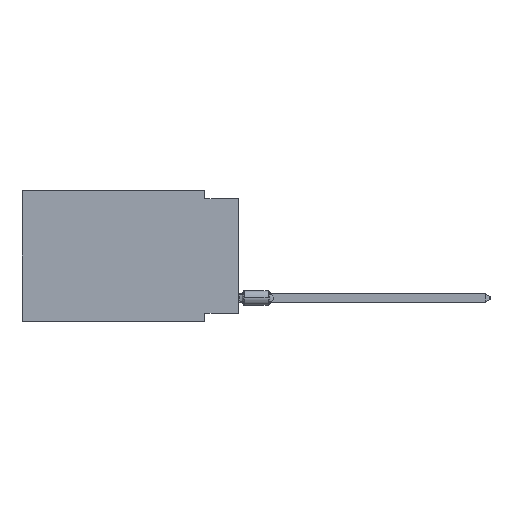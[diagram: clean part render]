
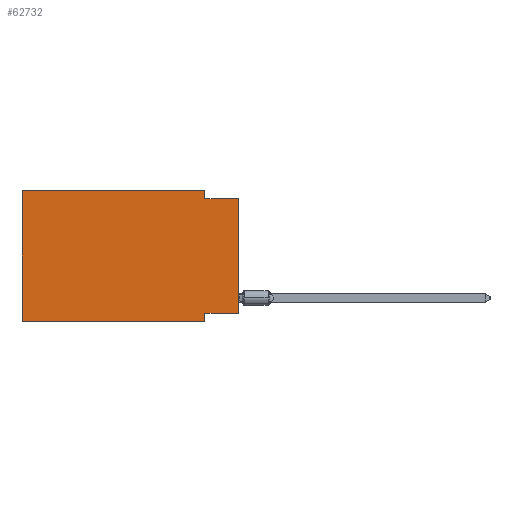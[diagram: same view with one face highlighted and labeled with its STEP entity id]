
A CAD part, left-side view. The second image highlights one B-rep face of the part: STEP entity #62732.
In plain terms, the highlighted planar face has unit normal (-1, 0, 0).
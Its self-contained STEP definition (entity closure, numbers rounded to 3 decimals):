
#473 = ORIENTED_EDGE ( 'NONE', *, *, #65297, .F. ) ;
#792 = CARTESIAN_POINT ( 'NONE',  ( 0., 0., -9.271 ) ) ;
#1288 = VERTEX_POINT ( 'NONE', #24832 ) ;
#1534 = ORIENTED_EDGE ( 'NONE', *, *, #37827, .F. ) ;
#1687 = VERTEX_POINT ( 'NONE', #4763 ) ;
#1880 = DIRECTION ( 'NONE',  ( 0., 0., 1. ) ) ;
#2244 = DIRECTION ( 'NONE',  ( 0., 0., -1. ) ) ;
#4738 = DIRECTION ( 'NONE',  ( 0., -1., 0. ) ) ;
#4763 = CARTESIAN_POINT ( 'NONE',  ( 0., 2.54, -0.635 ) ) ;
#4782 = VERTEX_POINT ( 'NONE', #67174 ) ;
#5969 = ORIENTED_EDGE ( 'NONE', *, *, #32607, .T. ) ;
#6378 = EDGE_LOOP ( 'NONE', ( #5969, #16772, #473, #15447, #13723, #21417, #56265, #1534 ) ) ;
#6649 = CARTESIAN_POINT ( 'NONE',  ( 0., 2.54, -9.906 ) ) ;
#7434 = DIRECTION ( 'NONE',  ( 0., -1., 0. ) ) ;
#8665 = VECTOR ( 'NONE', #42548, 1000. ) ;
#11778 = CARTESIAN_POINT ( 'NONE',  ( 0., 16.383, 0. ) ) ;
#12164 = PLANE ( 'NONE',  #34855 ) ;
#13723 = ORIENTED_EDGE ( 'NONE', *, *, #46928, .F. ) ;
#15167 = VECTOR ( 'NONE', #37014, 1000. ) ;
#15447 = ORIENTED_EDGE ( 'NONE', *, *, #65070, .F. ) ;
#15484 = CARTESIAN_POINT ( 'NONE',  ( 0., 16.383, 0. ) ) ;
#16772 = ORIENTED_EDGE ( 'NONE', *, *, #66112, .F. ) ;
#18406 = CARTESIAN_POINT ( 'NONE',  ( 0., 0., -0.635 ) ) ;
#18511 = CARTESIAN_POINT ( 'NONE',  ( 0., 2.54, 0. ) ) ;
#18996 = LINE ( 'NONE', #29242, #35188 ) ;
#19746 = CARTESIAN_POINT ( 'NONE',  ( 0., 16.383, -9.906 ) ) ;
#20221 = VECTOR ( 'NONE', #29838, 1000. ) ;
#21287 = VECTOR ( 'NONE', #4738, 1000. ) ;
#21417 = ORIENTED_EDGE ( 'NONE', *, *, #29095, .T. ) ;
#22633 = DIRECTION ( 'NONE',  ( 0., 0., -1. ) ) ;
#24391 = VERTEX_POINT ( 'NONE', #53255 ) ;
#24832 = CARTESIAN_POINT ( 'NONE',  ( 0., 16.383, 0. ) ) ;
#25863 = VECTOR ( 'NONE', #7434, 1000. ) ;
#29095 = EDGE_CURVE ( 'NONE', #24391, #58233, #66915, .T. ) ;
#29242 = CARTESIAN_POINT ( 'NONE',  ( 0., 0., -9.271 ) ) ;
#29838 = DIRECTION ( 'NONE',  ( 0., -1., 0. ) ) ;
#32607 = EDGE_CURVE ( 'NONE', #60291, #63623, #62307, .T. ) ;
#34855 = AXIS2_PLACEMENT_3D ( 'NONE', #59305, #53158, #2244 ) ;
#35188 = VECTOR ( 'NONE', #67162, 1000. ) ;
#37014 = DIRECTION ( 'NONE',  ( 0., 0., 1. ) ) ;
#37079 = LINE ( 'NONE', #11778, #43969 ) ;
#37827 = EDGE_CURVE ( 'NONE', #60291, #51407, #18996, .T. ) ;
#42548 = DIRECTION ( 'NONE',  ( 0., 0., -1. ) ) ;
#43586 = FACE_OUTER_BOUND ( 'NONE', #6378, .T. ) ;
#43661 = CARTESIAN_POINT ( 'NONE',  ( 0., 0., -0.635 ) ) ;
#43969 = VECTOR ( 'NONE', #1880, 1000. ) ;
#46928 = EDGE_CURVE ( 'NONE', #24391, #1288, #37079, .T. ) ;
#49463 = LINE ( 'NONE', #43661, #25863 ) ;
#51407 = VERTEX_POINT ( 'NONE', #59390 ) ;
#52455 = LINE ( 'NONE', #57575, #8665 ) ;
#53158 = DIRECTION ( 'NONE',  ( 1., 0., 0. ) ) ;
#53255 = CARTESIAN_POINT ( 'NONE',  ( 0., 16.383, -9.906 ) ) ;
#56265 = ORIENTED_EDGE ( 'NONE', *, *, #67474, .F. ) ;
#57575 = CARTESIAN_POINT ( 'NONE',  ( 0., 2.54, -9.906 ) ) ;
#58233 = VERTEX_POINT ( 'NONE', #6649 ) ;
#59305 = CARTESIAN_POINT ( 'NONE',  ( 0., 16.383, 0. ) ) ;
#59390 = CARTESIAN_POINT ( 'NONE',  ( 0., 2.54, -9.271 ) ) ;
#60291 = VERTEX_POINT ( 'NONE', #792 ) ;
#62307 = LINE ( 'NONE', #67104, #15167 ) ;
#62732 = ADVANCED_FACE ( 'NONE', ( #43586 ), #12164, .F. ) ;
#63623 = VERTEX_POINT ( 'NONE', #18406 ) ;
#64339 = LINE ( 'NONE', #18511, #66085 ) ;
#65070 = EDGE_CURVE ( 'NONE', #1288, #4782, #66080, .T. ) ;
#65297 = EDGE_CURVE ( 'NONE', #4782, #1687, #64339, .T. ) ;
#66080 = LINE ( 'NONE', #15484, #20221 ) ;
#66085 = VECTOR ( 'NONE', #22633, 1000. ) ;
#66112 = EDGE_CURVE ( 'NONE', #1687, #63623, #49463, .T. ) ;
#66915 = LINE ( 'NONE', #19746, #21287 ) ;
#67104 = CARTESIAN_POINT ( 'NONE',  ( 0., 0., 0. ) ) ;
#67162 = DIRECTION ( 'NONE',  ( 0., 1., 0. ) ) ;
#67174 = CARTESIAN_POINT ( 'NONE',  ( 0., 2.54, 0. ) ) ;
#67474 = EDGE_CURVE ( 'NONE', #51407, #58233, #52455, .T. ) ;
